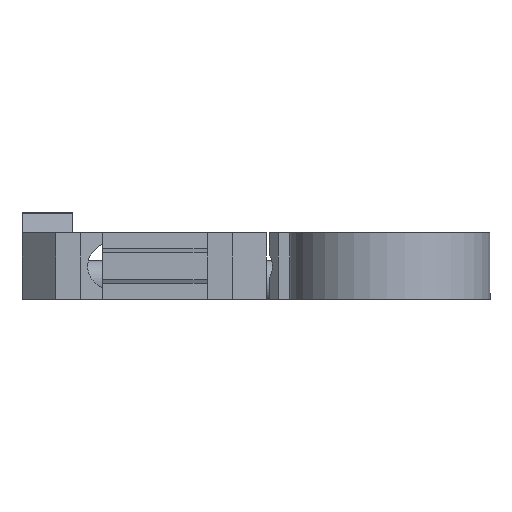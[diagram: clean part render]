
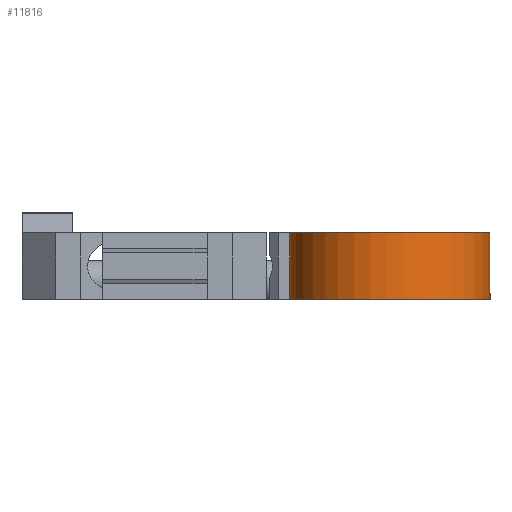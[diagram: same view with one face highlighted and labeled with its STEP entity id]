
A CAD part, front view. The second image highlights one B-rep face of the part: STEP entity #11816.
In plain terms, the highlighted cylindrical face has radius 15.24 mm (diameter 30.48 mm), a partial arc.
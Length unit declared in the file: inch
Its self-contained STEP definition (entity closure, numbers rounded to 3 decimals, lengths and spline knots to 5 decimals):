
#392 = EDGE_LOOP ( 'NONE', ( #2901, #2552, #1463, #4678 ) ) ;
#671 = CARTESIAN_POINT ( 'NONE',  ( 1.12297, -0.38462, -0.37124 ) ) ;
#673 = VERTEX_POINT ( 'NONE', #3174 ) ;
#716 = AXIS2_PLACEMENT_3D ( 'NONE', #11196, #8792, #14719 ) ;
#1232 = CARTESIAN_POINT ( 'NONE',  ( 1.53797, 0.04871, 1.67156 ) ) ;
#1463 = ORIENTED_EDGE ( 'NONE', *, *, #9734, .T. ) ;
#1483 = AXIS2_PLACEMENT_3D ( 'NONE', #671, #3163, #5571 ) ;
#2552 = ORIENTED_EDGE ( 'NONE', *, *, #8898, .T. ) ;
#2761 = CIRCLE ( 'NONE', #1483, 0.6 ) ;
#2901 = ORIENTED_EDGE ( 'NONE', *, *, #6512, .T. ) ;
#3163 = DIRECTION ( 'NONE',  ( 0., 0., -1. ) ) ;
#3174 = CARTESIAN_POINT ( 'NONE',  ( 1.53797, 0.04871, -0.77124 ) ) ;
#3904 = VECTOR ( 'NONE', #15348, 39.37008 ) ;
#4678 = ORIENTED_EDGE ( 'NONE', *, *, #14677, .T. ) ;
#4774 = VERTEX_POINT ( 'NONE', #6446 ) ;
#5017 = LINE ( 'NONE', #1232, #3904 ) ;
#5200 = DIRECTION ( 'NONE',  ( 0., 0., -1. ) ) ;
#5567 = AXIS2_PLACEMENT_3D ( 'NONE', #8902, #14821, #8949 ) ;
#5571 = DIRECTION ( 'NONE',  ( -1., 0., 0. ) ) ;
#6446 = CARTESIAN_POINT ( 'NONE',  ( 1.53797, 0.04871, -0.37124 ) ) ;
#6512 = EDGE_CURVE ( 'NONE', #4774, #13736, #2761, .T. ) ;
#7485 = VERTEX_POINT ( 'NONE', #11654 ) ;
#8792 = DIRECTION ( 'NONE',  ( 0., 0., 1. ) ) ;
#8898 = EDGE_CURVE ( 'NONE', #13736, #7485, #9005, .T. ) ;
#8902 = CARTESIAN_POINT ( 'NONE',  ( 1.12297, -0.38462, 1.67156 ) ) ;
#8949 = DIRECTION ( 'NONE',  ( -1., 0., 0. ) ) ;
#9005 = LINE ( 'NONE', #11207, #9916 ) ;
#9734 = EDGE_CURVE ( 'NONE', #7485, #673, #10288, .T. ) ;
#9916 = VECTOR ( 'NONE', #5200, 39.37008 ) ;
#10288 = CIRCLE ( 'NONE', #716, 0.6 ) ;
#11196 = CARTESIAN_POINT ( 'NONE',  ( 1.12297, -0.38462, -0.77124 ) ) ;
#11207 = CARTESIAN_POINT ( 'NONE',  ( 0.52297, -0.38462, 1.67156 ) ) ;
#11654 = CARTESIAN_POINT ( 'NONE',  ( 0.52297, -0.38462, -0.77124 ) ) ;
#11816 = ADVANCED_FACE ( 'NONE', ( #13219 ), #12114, .T. ) ;
#12114 = CYLINDRICAL_SURFACE ( 'NONE', #5567, 0.6 ) ;
#13219 = FACE_OUTER_BOUND ( 'NONE', #392, .T. ) ;
#13465 = CARTESIAN_POINT ( 'NONE',  ( 0.52297, -0.38462, -0.37124 ) ) ;
#13736 = VERTEX_POINT ( 'NONE', #13465 ) ;
#14677 = EDGE_CURVE ( 'NONE', #673, #4774, #5017, .T. ) ;
#14719 = DIRECTION ( 'NONE',  ( 1., 0., 0. ) ) ;
#14821 = DIRECTION ( 'NONE',  ( 0., 0., -1. ) ) ;
#15348 = DIRECTION ( 'NONE',  ( 0., 0., 1. ) ) ;
